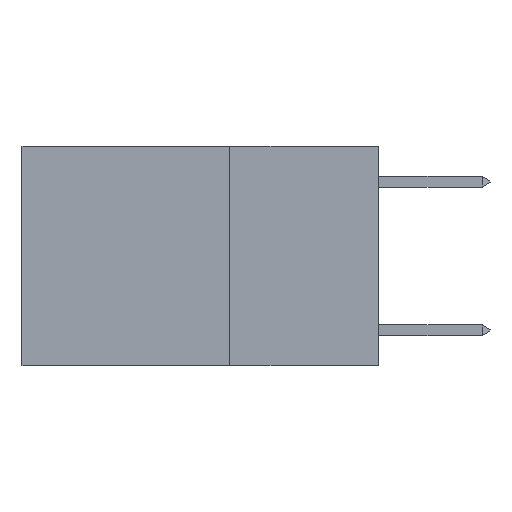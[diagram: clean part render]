
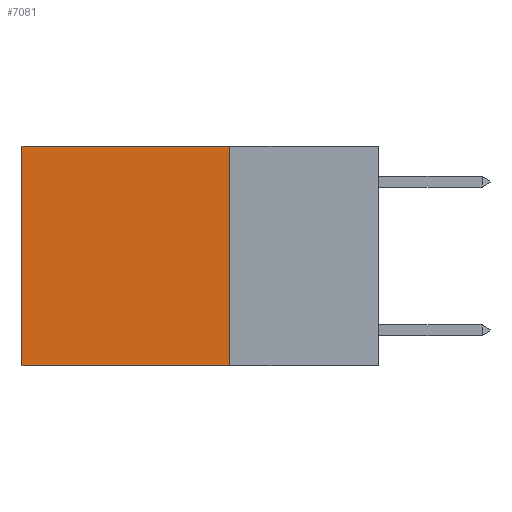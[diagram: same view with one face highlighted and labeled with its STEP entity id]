
A CAD part, left-side view. The second image highlights one B-rep face of the part: STEP entity #7081.
In plain terms, the highlighted planar face has unit normal (-1, 0, 0).
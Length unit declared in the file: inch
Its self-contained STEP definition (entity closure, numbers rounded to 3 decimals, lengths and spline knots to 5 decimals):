
#567 = DIRECTION ( 'NONE',  ( 0., 1., 0. ) ) ;
#595 = DIRECTION ( 'NONE',  ( 0., 1., 0. ) ) ;
#819 = VECTOR ( 'NONE', #3632, 39.37008 ) ;
#1090 = CARTESIAN_POINT ( 'NONE',  ( 0.2625, 0.6, -0.37 ) ) ;
#1432 = ORIENTED_EDGE ( 'NONE', *, *, #3672, .T. ) ;
#1454 = DIRECTION ( 'NONE',  ( 1., 0., 0. ) ) ;
#1550 = EDGE_LOOP ( 'NONE', ( #1432, #6137, #8533, #3712 ) ) ;
#2157 = CARTESIAN_POINT ( 'NONE',  ( 0.2625, 0.25, 0. ) ) ;
#2851 = CARTESIAN_POINT ( 'NONE',  ( 0.2625, 0.25, 0. ) ) ;
#2960 = DIRECTION ( 'NONE',  ( 0., 0., -1. ) ) ;
#3632 = DIRECTION ( 'NONE',  ( 0., 0., -1. ) ) ;
#3661 = VERTEX_POINT ( 'NONE', #6288 ) ;
#3672 = EDGE_CURVE ( 'NONE', #9949, #9620, #6232, .T. ) ;
#3712 = ORIENTED_EDGE ( 'NONE', *, *, #10771, .T. ) ;
#4476 = CARTESIAN_POINT ( 'NONE',  ( 0.2625, 0.25, 0. ) ) ;
#4554 = VECTOR ( 'NONE', #2960, 39.37008 ) ;
#4639 = CARTESIAN_POINT ( 'NONE',  ( 0.2625, 0.6, 0. ) ) ;
#5518 = FACE_OUTER_BOUND ( 'NONE', #1550, .T. ) ;
#5611 = CARTESIAN_POINT ( 'NONE',  ( 0.2625, 0.25, -0.37 ) ) ;
#6137 = ORIENTED_EDGE ( 'NONE', *, *, #7588, .F. ) ;
#6232 = LINE ( 'NONE', #4639, #4554 ) ;
#6288 = CARTESIAN_POINT ( 'NONE',  ( 0.2625, 0.25, -0.37 ) ) ;
#6360 = LINE ( 'NONE', #2157, #10186 ) ;
#6941 = LINE ( 'NONE', #2851, #819 ) ;
#7081 = ADVANCED_FACE ( 'NONE', ( #5518 ), #10493, .F. ) ;
#7154 = LINE ( 'NONE', #5611, #7304 ) ;
#7229 = CARTESIAN_POINT ( 'NONE',  ( 0.2625, 0.25, 0. ) ) ;
#7304 = VECTOR ( 'NONE', #567, 39.37008 ) ;
#7398 = EDGE_CURVE ( 'NONE', #10126, #3661, #6941, .T. ) ;
#7588 = EDGE_CURVE ( 'NONE', #3661, #9620, #7154, .T. ) ;
#7790 = CARTESIAN_POINT ( 'NONE',  ( 0.2625, 0.6, 0. ) ) ;
#8104 = DIRECTION ( 'NONE',  ( 0., 0., -1. ) ) ;
#8533 = ORIENTED_EDGE ( 'NONE', *, *, #7398, .F. ) ;
#9620 = VERTEX_POINT ( 'NONE', #1090 ) ;
#9949 = VERTEX_POINT ( 'NONE', #7790 ) ;
#10126 = VERTEX_POINT ( 'NONE', #4476 ) ;
#10186 = VECTOR ( 'NONE', #595, 39.37008 ) ;
#10493 = PLANE ( 'NONE',  #10662 ) ;
#10662 = AXIS2_PLACEMENT_3D ( 'NONE', #7229, #1454, #8104 ) ;
#10771 = EDGE_CURVE ( 'NONE', #10126, #9949, #6360, .T. ) ;
